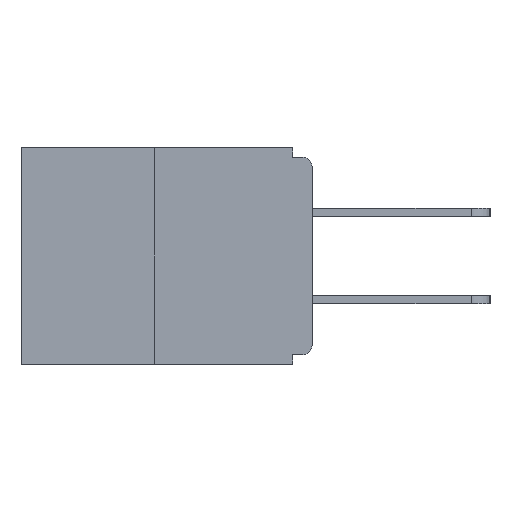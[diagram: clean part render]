
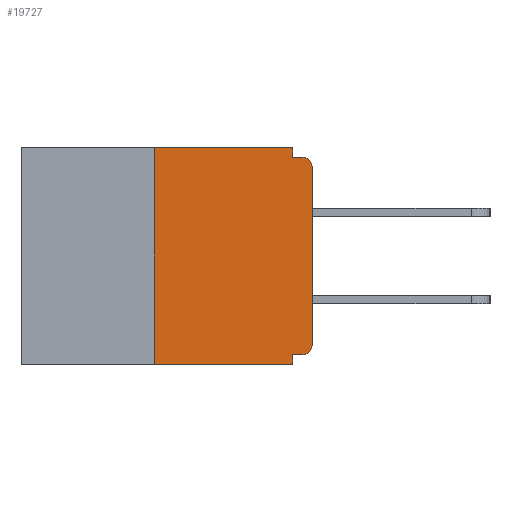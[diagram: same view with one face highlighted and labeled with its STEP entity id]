
A CAD part, left-side view. The second image highlights one B-rep face of the part: STEP entity #19727.
In plain terms, the highlighted planar face has unit normal (-1, 0, 0).
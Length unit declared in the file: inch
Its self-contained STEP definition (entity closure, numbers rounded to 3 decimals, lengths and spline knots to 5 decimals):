
#10 = CARTESIAN_POINT ( 'NONE',  ( 0., 0., -0.03 ) ) ;
#68 = VECTOR ( 'NONE', #1387, 39.37008 ) ;
#491 = ORIENTED_EDGE ( 'NONE', *, *, #6490, .T. ) ;
#800 = DIRECTION ( 'NONE',  ( 0., 0., 1. ) ) ;
#1387 = DIRECTION ( 'NONE',  ( 0., 0., 1. ) ) ;
#1509 = CARTESIAN_POINT ( 'NONE',  ( 0., 0.015, -0.313 ) ) ;
#1778 = ORIENTED_EDGE ( 'NONE', *, *, #26425, .F. ) ;
#2876 = CARTESIAN_POINT ( 'NONE',  ( 0., 0., -0.313 ) ) ;
#2935 = ORIENTED_EDGE ( 'NONE', *, *, #17289, .F. ) ;
#3188 = VERTEX_POINT ( 'NONE', #8605 ) ;
#3588 = DIRECTION ( 'NONE',  ( -1., 0., 0. ) ) ;
#3722 = LINE ( 'NONE', #4856, #15426 ) ;
#3838 = CIRCLE ( 'NONE', #29929, 0.015 ) ;
#3941 = VECTOR ( 'NONE', #800, 39.37008 ) ;
#4601 = VERTEX_POINT ( 'NONE', #9868 ) ;
#4856 = CARTESIAN_POINT ( 'NONE',  ( 0., 0.031, -0.343 ) ) ;
#5282 = CARTESIAN_POINT ( 'NONE',  ( 0., 0.031, -0.343 ) ) ;
#5481 = AXIS2_PLACEMENT_3D ( 'NONE', #23068, #18143, #8973 ) ;
#5629 = VERTEX_POINT ( 'NONE', #29585 ) ;
#5667 = DIRECTION ( 'NONE',  ( 0., 0., -1. ) ) ;
#5777 = CARTESIAN_POINT ( 'NONE',  ( 0., 0.031, 0. ) ) ;
#5918 = CARTESIAN_POINT ( 'NONE',  ( 0., 0., 0. ) ) ;
#6155 = LINE ( 'NONE', #19360, #3941 ) ;
#6346 = LINE ( 'NONE', #5918, #68 ) ;
#6490 = EDGE_CURVE ( 'NONE', #5629, #13311, #25380, .T. ) ;
#7878 = CARTESIAN_POINT ( 'NONE',  ( 0., 0.46, -0.343 ) ) ;
#8412 = DIRECTION ( 'NONE',  ( 0., 0., -1. ) ) ;
#8605 = CARTESIAN_POINT ( 'NONE',  ( 0., 0.015, -0.015 ) ) ;
#8973 = DIRECTION ( 'NONE',  ( 0., 0., -1. ) ) ;
#9727 = VERTEX_POINT ( 'NONE', #10 ) ;
#9868 = CARTESIAN_POINT ( 'NONE',  ( 0., 0.015, -0.328 ) ) ;
#10001 = ORIENTED_EDGE ( 'NONE', *, *, #16239, .F. ) ;
#10677 = CARTESIAN_POINT ( 'NONE',  ( 0., 0.031, 0. ) ) ;
#10877 = EDGE_CURVE ( 'NONE', #5629, #29536, #6155, .T. ) ;
#11877 = VERTEX_POINT ( 'NONE', #27449 ) ;
#12033 = DIRECTION ( 'NONE',  ( 0., -1., 0. ) ) ;
#12361 = AXIS2_PLACEMENT_3D ( 'NONE', #28989, #26763, #5667 ) ;
#12740 = VECTOR ( 'NONE', #27048, 39.37008 ) ;
#13311 = VERTEX_POINT ( 'NONE', #5282 ) ;
#13474 = CIRCLE ( 'NONE', #12361, 0.015 ) ;
#14175 = LINE ( 'NONE', #16422, #25862 ) ;
#14949 = EDGE_CURVE ( 'NONE', #22623, #28970, #27946, .T. ) ;
#15049 = DIRECTION ( 'NONE',  ( 0., -1., 0. ) ) ;
#15105 = VECTOR ( 'NONE', #15049, 39.37008 ) ;
#15426 = VECTOR ( 'NONE', #21330, 39.37008 ) ;
#15634 = FACE_OUTER_BOUND ( 'NONE', #27162, .T. ) ;
#16077 = VECTOR ( 'NONE', #28255, 39.37008 ) ;
#16239 = EDGE_CURVE ( 'NONE', #11877, #13311, #3722, .T. ) ;
#16422 = CARTESIAN_POINT ( 'NONE',  ( 0., 0., -0.015 ) ) ;
#16601 = VERTEX_POINT ( 'NONE', #2876 ) ;
#17289 = EDGE_CURVE ( 'NONE', #29536, #22623, #18289, .T. ) ;
#18143 = DIRECTION ( 'NONE',  ( 1., 0., 0. ) ) ;
#18289 = LINE ( 'NONE', #25920, #16077 ) ;
#18310 = ORIENTED_EDGE ( 'NONE', *, *, #29039, .T. ) ;
#18594 = LINE ( 'NONE', #20294, #12740 ) ;
#19360 = CARTESIAN_POINT ( 'NONE',  ( 0., 0.25, 0. ) ) ;
#19432 = EDGE_CURVE ( 'NONE', #9727, #3188, #13474, .T. ) ;
#19575 = EDGE_CURVE ( 'NONE', #4601, #11877, #18594, .T. ) ;
#19727 = ADVANCED_FACE ( 'NONE', ( #15634 ), #30114, .F. ) ;
#20294 = CARTESIAN_POINT ( 'NONE',  ( 0., 0., -0.328 ) ) ;
#20849 = ORIENTED_EDGE ( 'NONE', *, *, #19575, .F. ) ;
#21330 = DIRECTION ( 'NONE',  ( 0., 0., -1. ) ) ;
#22584 = ORIENTED_EDGE ( 'NONE', *, *, #14949, .F. ) ;
#22623 = VERTEX_POINT ( 'NONE', #10677 ) ;
#23068 = CARTESIAN_POINT ( 'NONE',  ( 0., 0.46, 0. ) ) ;
#23173 = ORIENTED_EDGE ( 'NONE', *, *, #10877, .F. ) ;
#24815 = DIRECTION ( 'NONE',  ( 0., 0., -1. ) ) ;
#25380 = LINE ( 'NONE', #7878, #15105 ) ;
#25595 = EDGE_CURVE ( 'NONE', #4601, #16601, #3838, .T. ) ;
#25862 = VECTOR ( 'NONE', #12033, 39.37008 ) ;
#25920 = CARTESIAN_POINT ( 'NONE',  ( 0., 0.46, 0. ) ) ;
#26425 = EDGE_CURVE ( 'NONE', #28970, #3188, #14175, .T. ) ;
#26763 = DIRECTION ( 'NONE',  ( -1., 0., 0. ) ) ;
#26850 = ORIENTED_EDGE ( 'NONE', *, *, #19432, .T. ) ;
#26900 = CARTESIAN_POINT ( 'NONE',  ( 0., 0.031, -0.015 ) ) ;
#27048 = DIRECTION ( 'NONE',  ( 0., 1., 0. ) ) ;
#27162 = EDGE_LOOP ( 'NONE', ( #2935, #23173, #491, #10001, #20849, #28249, #18310, #26850, #1778, #22584 ) ) ;
#27209 = VECTOR ( 'NONE', #24815, 39.37008 ) ;
#27449 = CARTESIAN_POINT ( 'NONE',  ( 0., 0.031, -0.328 ) ) ;
#27946 = LINE ( 'NONE', #5777, #27209 ) ;
#28249 = ORIENTED_EDGE ( 'NONE', *, *, #25595, .T. ) ;
#28255 = DIRECTION ( 'NONE',  ( 0., -1., 0. ) ) ;
#28970 = VERTEX_POINT ( 'NONE', #26900 ) ;
#28989 = CARTESIAN_POINT ( 'NONE',  ( 0., 0.015, -0.03 ) ) ;
#29039 = EDGE_CURVE ( 'NONE', #16601, #9727, #6346, .T. ) ;
#29420 = CARTESIAN_POINT ( 'NONE',  ( 0., 0.25, 0. ) ) ;
#29536 = VERTEX_POINT ( 'NONE', #29420 ) ;
#29585 = CARTESIAN_POINT ( 'NONE',  ( 0., 0.25, -0.343 ) ) ;
#29929 = AXIS2_PLACEMENT_3D ( 'NONE', #1509, #3588, #8412 ) ;
#30114 = PLANE ( 'NONE',  #5481 ) ;
